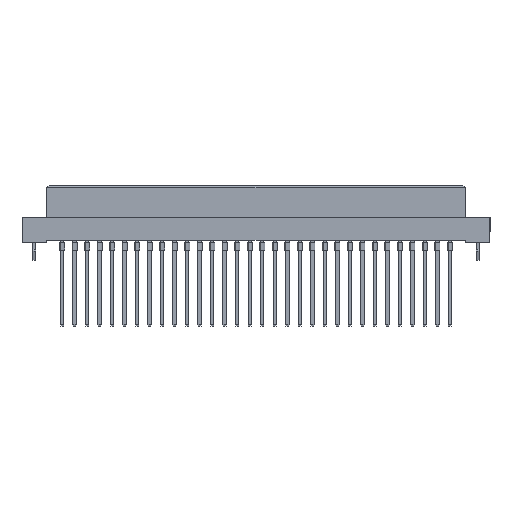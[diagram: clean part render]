
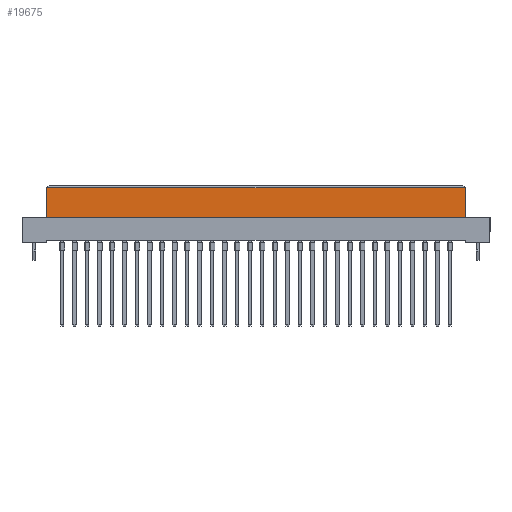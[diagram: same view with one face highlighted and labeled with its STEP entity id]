
A CAD part, top view. The second image highlights one B-rep face of the part: STEP entity #19675.
In plain terms, the highlighted planar face has unit normal (0, 0, 1).
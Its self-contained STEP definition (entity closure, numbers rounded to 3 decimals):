
#1629 = CARTESIAN_POINT ( 'NONE',  ( 42.5, -6.4, 4.25 ) ) ;
#4009 = ORIENTED_EDGE ( 'NONE', *, *, #16337, .T. ) ;
#4199 = CARTESIAN_POINT ( 'NONE',  ( -42.5, -6.4, 4.25 ) ) ;
#4319 = DIRECTION ( 'NONE',  ( 0., 1., 0. ) ) ;
#4324 = VECTOR ( 'NONE', #25354, 1000. ) ;
#8134 = CARTESIAN_POINT ( 'NONE',  ( 42.5, -6.4, 4.25 ) ) ;
#8657 = CARTESIAN_POINT ( 'NONE',  ( 42.5, -6.4, 4.25 ) ) ;
#10425 = DIRECTION ( 'NONE',  ( 0., 0., 1. ) ) ;
#11791 = CARTESIAN_POINT ( 'NONE',  ( -42.5, -6.4, 4.25 ) ) ;
#12379 = ORIENTED_EDGE ( 'NONE', *, *, #32751, .F. ) ;
#13601 = VECTOR ( 'NONE', #4319, 1000. ) ;
#16337 = EDGE_CURVE ( 'NONE', #35402, #20622, #29438, .T. ) ;
#19675 = ADVANCED_FACE ( 'NONE', ( #38643 ), #36354, .T. ) ;
#20511 = CARTESIAN_POINT ( 'NONE',  ( 42.5, -6.4, 4.25 ) ) ;
#20622 = VERTEX_POINT ( 'NONE', #20680 ) ;
#20680 = CARTESIAN_POINT ( 'NONE',  ( 42.5, -0.5, 4.25 ) ) ;
#23056 = CARTESIAN_POINT ( 'NONE',  ( -42.5, -0.5, 4.25 ) ) ;
#23942 = VECTOR ( 'NONE', #33820, 1000. ) ;
#25270 = ORIENTED_EDGE ( 'NONE', *, *, #33321, .T. ) ;
#25282 = VECTOR ( 'NONE', #26280, 1000. ) ;
#25354 = DIRECTION ( 'NONE',  ( -1., 0., 0. ) ) ;
#25749 = LINE ( 'NONE', #40585, #4324 ) ;
#26025 = VERTEX_POINT ( 'NONE', #23056 ) ;
#26280 = DIRECTION ( 'NONE',  ( 1., 0., 0. ) ) ;
#26998 = ORIENTED_EDGE ( 'NONE', *, *, #36919, .T. ) ;
#27030 = LINE ( 'NONE', #11791, #23942 ) ;
#29438 = LINE ( 'NONE', #1629, #13601 ) ;
#32443 = DIRECTION ( 'NONE',  ( 1., 0., 0. ) ) ;
#32751 = EDGE_CURVE ( 'NONE', #33761, #26025, #27030, .T. ) ;
#33155 = AXIS2_PLACEMENT_3D ( 'NONE', #8134, #10425, #32443 ) ;
#33321 = EDGE_CURVE ( 'NONE', #33761, #35402, #36359, .T. ) ;
#33761 = VERTEX_POINT ( 'NONE', #4199 ) ;
#33820 = DIRECTION ( 'NONE',  ( 0., 1., 0. ) ) ;
#35402 = VERTEX_POINT ( 'NONE', #8657 ) ;
#36354 = PLANE ( 'NONE',  #33155 ) ;
#36359 = LINE ( 'NONE', #20511, #25282 ) ;
#36919 = EDGE_CURVE ( 'NONE', #20622, #26025, #25749, .T. ) ;
#38643 = FACE_OUTER_BOUND ( 'NONE', #39319, .T. ) ;
#39319 = EDGE_LOOP ( 'NONE', ( #4009, #26998, #12379, #25270 ) ) ;
#40585 = CARTESIAN_POINT ( 'NONE',  ( -42.5, -0.5, 4.25 ) ) ;
